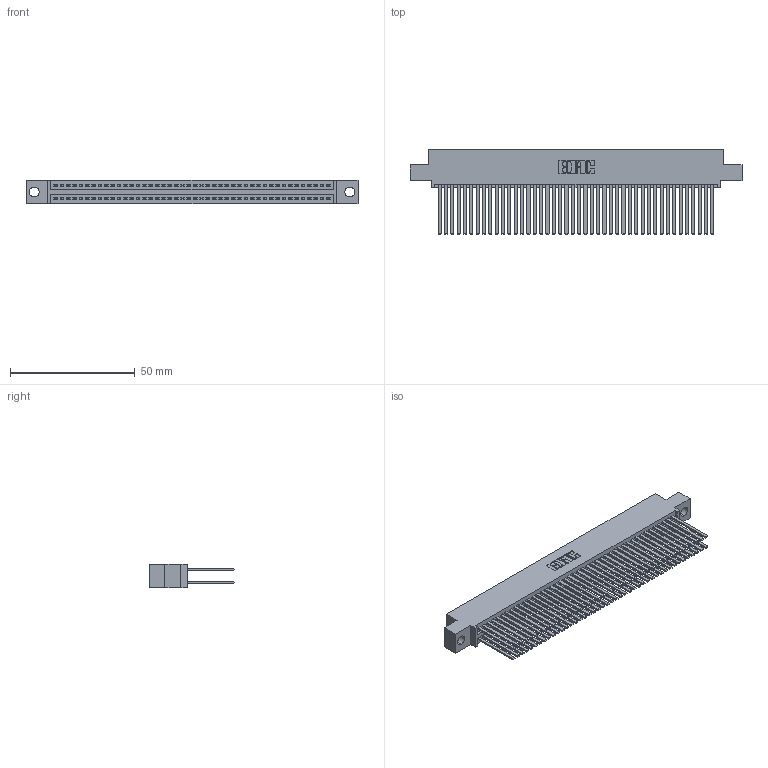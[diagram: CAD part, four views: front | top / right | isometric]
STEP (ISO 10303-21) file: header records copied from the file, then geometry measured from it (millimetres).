
FILE_DESCRIPTION (( 'STEP AP203' ), '1' );
FILE_NAME ('395-088-544-504.STEP', '2021-06-17T09:36:56', ( '' ), ( '' ), 'SwSTEP 2.0', 'SolidWorks 2020', '' );
FILE_SCHEMA (( 'CONFIG_CONTROL_DESIGN' ));
Length unit declared in the file: inch
Products named in the file (3): 345-292-001_345-293-144; 345 Part_0.110 Offset - 0.156 Dia-TI; 395-088-544-504
Assembly tree (89 placements, depth 2):
  395-088-544-504
    345 Part_0.110 Offset - 0.156 Dia-TI
    345-292-001_345-293-144  x88
Bounding box: 132.97 x 33.96 x 9.4 mm (x, y, z)
Volume: 13989.6 mm3; surface area: 24277.7 mm2
Topology: 89 solids, 89 shells, 4016 faces, 11917 edges, 7826 vertices
Faces by surface type: plane 2650, cylinder 1366
Entity records: 34621 total; most frequent: CARTESIAN_POINT 5806, ORIENTED_EDGE 5738, DIRECTION 5113, EDGE_CURVE 2869, VECTOR 2565, LINE 2565, VERTEX_POINT 1910, AXIS2_PLACEMENT_3D 1274
